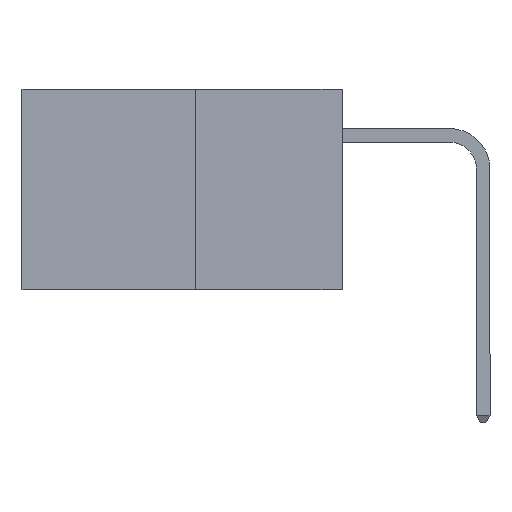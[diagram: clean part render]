
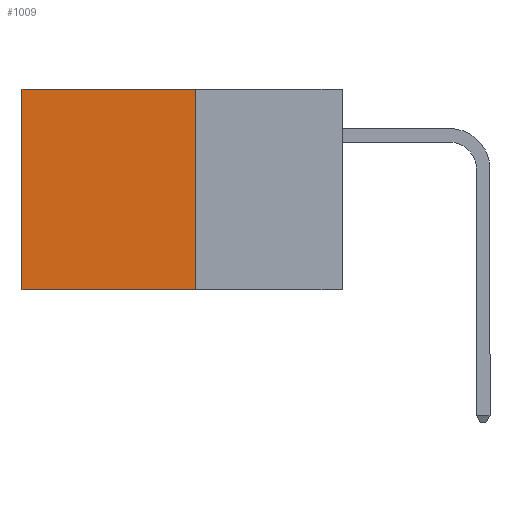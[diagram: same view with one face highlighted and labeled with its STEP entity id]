
A CAD part, left-side view. The second image highlights one B-rep face of the part: STEP entity #1009.
In plain terms, the highlighted planar face has unit normal (-1, 0, 0).
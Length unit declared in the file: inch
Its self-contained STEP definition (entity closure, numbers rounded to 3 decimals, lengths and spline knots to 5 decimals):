
#551 = FACE_OUTER_BOUND ( 'NONE', #6475, .T. ) ;
#771 = EDGE_CURVE ( 'NONE', #3991, #12843, #9311, .T. ) ;
#847 = ORIENTED_EDGE ( 'NONE', *, *, #9043, .F. ) ;
#928 = DIRECTION ( 'NONE',  ( 0., 0., -1. ) ) ;
#1009 = ADVANCED_FACE ( 'NONE', ( #551 ), #9037, .F. ) ;
#3185 = CARTESIAN_POINT ( 'NONE',  ( 0.277, 0.59, -0.37 ) ) ;
#3991 = VERTEX_POINT ( 'NONE', #4469 ) ;
#4098 = ORIENTED_EDGE ( 'NONE', *, *, #7794, .T. ) ;
#4248 = CARTESIAN_POINT ( 'NONE',  ( 0.277, 0.27, -0.37 ) ) ;
#4281 = DIRECTION ( 'NONE',  ( 0., 1., 0. ) ) ;
#4469 = CARTESIAN_POINT ( 'NONE',  ( 0.277, 0.59, 0. ) ) ;
#5736 = AXIS2_PLACEMENT_3D ( 'NONE', #7323, #13187, #928 ) ;
#6277 = LINE ( 'NONE', #4248, #14139 ) ;
#6475 = EDGE_LOOP ( 'NONE', ( #6810, #9741, #847, #4098 ) ) ;
#6810 = ORIENTED_EDGE ( 'NONE', *, *, #771, .T. ) ;
#7197 = VERTEX_POINT ( 'NONE', #13547 ) ;
#7323 = CARTESIAN_POINT ( 'NONE',  ( 0.277, 0.27, -0.37 ) ) ;
#7441 = DIRECTION ( 'NONE',  ( 0., 0., -1. ) ) ;
#7794 = EDGE_CURVE ( 'NONE', #9055, #3991, #11576, .T. ) ;
#8330 = VECTOR ( 'NONE', #13450, 39.37008 ) ;
#8365 = VECTOR ( 'NONE', #8743, 39.37008 ) ;
#8404 = EDGE_CURVE ( 'NONE', #7197, #12843, #6277, .T. ) ;
#8613 = CARTESIAN_POINT ( 'NONE',  ( 0.277, 0.27, 0. ) ) ;
#8743 = DIRECTION ( 'NONE',  ( 0., 1., 0. ) ) ;
#8956 = VECTOR ( 'NONE', #7441, 39.37008 ) ;
#9037 = PLANE ( 'NONE',  #5736 ) ;
#9043 = EDGE_CURVE ( 'NONE', #9055, #7197, #11531, .T. ) ;
#9055 = VERTEX_POINT ( 'NONE', #13797 ) ;
#9311 = LINE ( 'NONE', #3185, #8956 ) ;
#9741 = ORIENTED_EDGE ( 'NONE', *, *, #8404, .F. ) ;
#11531 = LINE ( 'NONE', #13874, #8330 ) ;
#11576 = LINE ( 'NONE', #8613, #8365 ) ;
#12738 = CARTESIAN_POINT ( 'NONE',  ( 0.277, 0.59, -0.37 ) ) ;
#12843 = VERTEX_POINT ( 'NONE', #12738 ) ;
#13187 = DIRECTION ( 'NONE',  ( 1., 0., 0. ) ) ;
#13450 = DIRECTION ( 'NONE',  ( 0., 0., -1. ) ) ;
#13547 = CARTESIAN_POINT ( 'NONE',  ( 0.277, 0.27, -0.37 ) ) ;
#13797 = CARTESIAN_POINT ( 'NONE',  ( 0.277, 0.27, 0. ) ) ;
#13874 = CARTESIAN_POINT ( 'NONE',  ( 0.277, 0.27, -0.37 ) ) ;
#14139 = VECTOR ( 'NONE', #4281, 39.37008 ) ;
